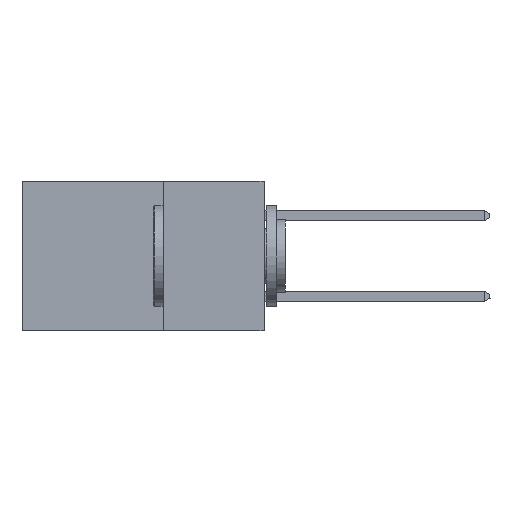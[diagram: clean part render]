
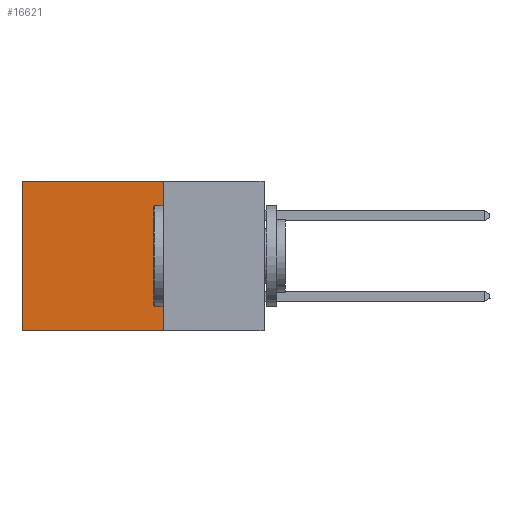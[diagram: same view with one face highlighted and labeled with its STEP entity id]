
A CAD part, left-side view. The second image highlights one B-rep face of the part: STEP entity #16621.
In plain terms, the highlighted planar face has unit normal (-1, 0, 0).
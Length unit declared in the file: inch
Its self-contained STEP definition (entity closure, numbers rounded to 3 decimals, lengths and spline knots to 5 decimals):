
#356 = CARTESIAN_POINT ( 'NONE',  ( 0.2615, 0.6, -0.37 ) ) ;
#387 = LINE ( 'NONE', #17562, #17136 ) ;
#554 = CARTESIAN_POINT ( 'NONE',  ( 0.2615, 0.25, -0.37 ) ) ;
#862 = DIRECTION ( 'NONE',  ( 0., 1., 0. ) ) ;
#1876 = CARTESIAN_POINT ( 'NONE',  ( 0.2615, 0.25, 0. ) ) ;
#3717 = LINE ( 'NONE', #6893, #25543 ) ;
#4356 = AXIS2_PLACEMENT_3D ( 'NONE', #12902, #28150, #15106 ) ;
#5092 = FACE_OUTER_BOUND ( 'NONE', #26624, .T. ) ;
#6564 = CARTESIAN_POINT ( 'NONE',  ( 0.2615, 0.25, -0.37 ) ) ;
#6743 = EDGE_CURVE ( 'NONE', #13987, #22911, #387, .T. ) ;
#6853 = EDGE_CURVE ( 'NONE', #10821, #13987, #7877, .T. ) ;
#6893 = CARTESIAN_POINT ( 'NONE',  ( 0.2615, 0.6, -0.37 ) ) ;
#7644 = ORIENTED_EDGE ( 'NONE', *, *, #6743, .F. ) ;
#7877 = LINE ( 'NONE', #554, #15066 ) ;
#8497 = PLANE ( 'NONE',  #4356 ) ;
#9457 = ORIENTED_EDGE ( 'NONE', *, *, #17167, .T. ) ;
#9458 = CARTESIAN_POINT ( 'NONE',  ( 0.2615, 0.25, 0. ) ) ;
#10821 = VERTEX_POINT ( 'NONE', #1876 ) ;
#11156 = CARTESIAN_POINT ( 'NONE',  ( 0.2615, 0.6, 0. ) ) ;
#11207 = EDGE_CURVE ( 'NONE', #10821, #17132, #24451, .T. ) ;
#12902 = CARTESIAN_POINT ( 'NONE',  ( 0.2615, 0.25, -0.37 ) ) ;
#13485 = DIRECTION ( 'NONE',  ( 0., 0., -1. ) ) ;
#13987 = VERTEX_POINT ( 'NONE', #6564 ) ;
#15066 = VECTOR ( 'NONE', #15820, 39.37008 ) ;
#15106 = DIRECTION ( 'NONE',  ( 0., 0., -1. ) ) ;
#15820 = DIRECTION ( 'NONE',  ( 0., 0., -1. ) ) ;
#16621 = ADVANCED_FACE ( 'NONE', ( #5092 ), #8497, .F. ) ;
#17132 = VERTEX_POINT ( 'NONE', #11156 ) ;
#17136 = VECTOR ( 'NONE', #24079, 39.37008 ) ;
#17167 = EDGE_CURVE ( 'NONE', #17132, #22911, #3717, .T. ) ;
#17562 = CARTESIAN_POINT ( 'NONE',  ( 0.2615, 0.25, -0.37 ) ) ;
#19600 = ORIENTED_EDGE ( 'NONE', *, *, #6853, .F. ) ;
#22911 = VERTEX_POINT ( 'NONE', #356 ) ;
#23770 = VECTOR ( 'NONE', #862, 39.37008 ) ;
#23979 = ORIENTED_EDGE ( 'NONE', *, *, #11207, .T. ) ;
#24079 = DIRECTION ( 'NONE',  ( 0., 1., 0. ) ) ;
#24451 = LINE ( 'NONE', #9458, #23770 ) ;
#25543 = VECTOR ( 'NONE', #13485, 39.37008 ) ;
#26624 = EDGE_LOOP ( 'NONE', ( #9457, #7644, #19600, #23979 ) ) ;
#28150 = DIRECTION ( 'NONE',  ( 1., 0., 0. ) ) ;
